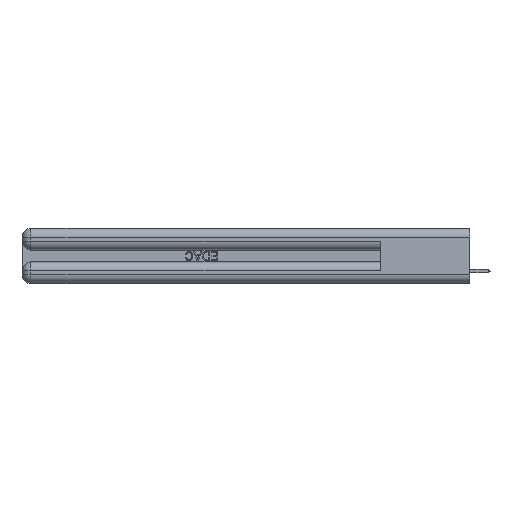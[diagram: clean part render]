
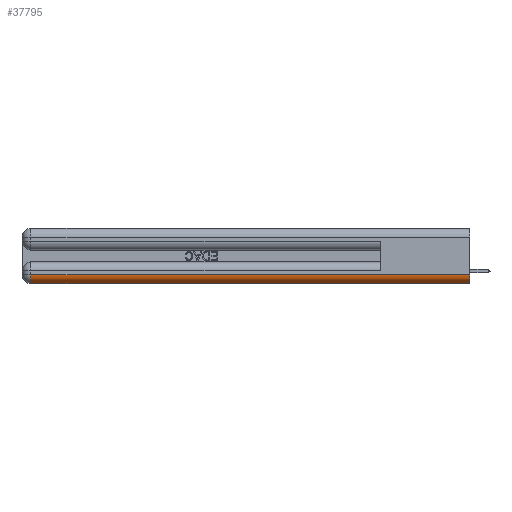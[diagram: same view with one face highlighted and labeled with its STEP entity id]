
A CAD part, left-side view. The second image highlights one B-rep face of the part: STEP entity #37795.
In plain terms, the highlighted cylindrical face has radius 1.524 mm (diameter 3.048 mm), a partial arc.
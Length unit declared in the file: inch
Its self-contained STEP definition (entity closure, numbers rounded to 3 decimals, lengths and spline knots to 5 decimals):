
#1167 = DIRECTION ( 'NONE',  ( 0., 1., 0. ) ) ;
#2231 = LINE ( 'NONE', #10518, #36931 ) ;
#2906 = VERTEX_POINT ( 'NONE', #11616 ) ;
#3620 = DIRECTION ( 'NONE',  ( 0., 0., 1. ) ) ;
#3952 = DIRECTION ( 'NONE',  ( 0., -1., 0. ) ) ;
#5598 = EDGE_LOOP ( 'NONE', ( #32639, #43106, #35323, #41914 ) ) ;
#6079 = CARTESIAN_POINT ( 'NONE',  ( 0.06, 0., 0.06 ) ) ;
#6359 = DIRECTION ( 'NONE',  ( 0., 0., 1. ) ) ;
#6438 = LINE ( 'NONE', #13147, #41181 ) ;
#6548 = DIRECTION ( 'NONE',  ( 0., 1., 0. ) ) ;
#9046 = FACE_OUTER_BOUND ( 'NONE', #5598, .T. ) ;
#9713 = DIRECTION ( 'NONE',  ( 0., -1., 0. ) ) ;
#10518 = CARTESIAN_POINT ( 'NONE',  ( 0., 0., 0.06 ) ) ;
#11616 = CARTESIAN_POINT ( 'NONE',  ( 0., 2.94, 0.06 ) ) ;
#13147 = CARTESIAN_POINT ( 'NONE',  ( 0.06, 3., 0. ) ) ;
#13639 = EDGE_CURVE ( 'NONE', #2906, #26009, #2231, .T. ) ;
#14148 = AXIS2_PLACEMENT_3D ( 'NONE', #28169, #1167, #34803 ) ;
#18032 = CARTESIAN_POINT ( 'NONE',  ( 0.06, 0., 0. ) ) ;
#18520 = VERTEX_POINT ( 'NONE', #26679 ) ;
#19557 = EDGE_CURVE ( 'NONE', #28880, #18520, #6438, .T. ) ;
#25434 = AXIS2_PLACEMENT_3D ( 'NONE', #6079, #9713, #6359 ) ;
#26009 = VERTEX_POINT ( 'NONE', #38327 ) ;
#26679 = CARTESIAN_POINT ( 'NONE',  ( 0.06, 2.94, 0. ) ) ;
#28169 = CARTESIAN_POINT ( 'NONE',  ( 0.06, 2.94, 0.06 ) ) ;
#28880 = VERTEX_POINT ( 'NONE', #18032 ) ;
#29772 = EDGE_CURVE ( 'NONE', #26009, #28880, #31154, .T. ) ;
#31154 = CIRCLE ( 'NONE', #25434, 0.06 ) ;
#32639 = ORIENTED_EDGE ( 'NONE', *, *, #29772, .F. ) ;
#33725 = CIRCLE ( 'NONE', #14148, 0.06 ) ;
#33743 = CYLINDRICAL_SURFACE ( 'NONE', #39521, 0.06 ) ;
#34803 = DIRECTION ( 'NONE',  ( 0., 0., 1. ) ) ;
#35323 = ORIENTED_EDGE ( 'NONE', *, *, #40738, .F. ) ;
#36819 = CARTESIAN_POINT ( 'NONE',  ( 0.06, 0., 0.06 ) ) ;
#36931 = VECTOR ( 'NONE', #3952, 39.37008 ) ;
#37795 = ADVANCED_FACE ( 'NONE', ( #9046 ), #33743, .T. ) ;
#38327 = CARTESIAN_POINT ( 'NONE',  ( 0., 0., 0.06 ) ) ;
#39521 = AXIS2_PLACEMENT_3D ( 'NONE', #36819, #40391, #3620 ) ;
#40391 = DIRECTION ( 'NONE',  ( 0., 1., 0. ) ) ;
#40738 = EDGE_CURVE ( 'NONE', #18520, #2906, #33725, .T. ) ;
#41181 = VECTOR ( 'NONE', #6548, 39.37008 ) ;
#41914 = ORIENTED_EDGE ( 'NONE', *, *, #19557, .F. ) ;
#43106 = ORIENTED_EDGE ( 'NONE', *, *, #13639, .F. ) ;
